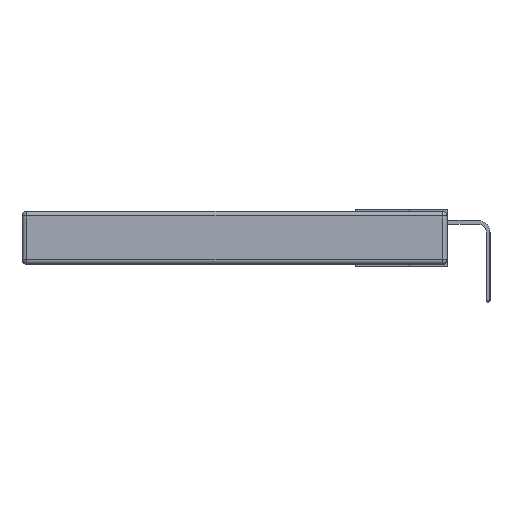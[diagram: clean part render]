
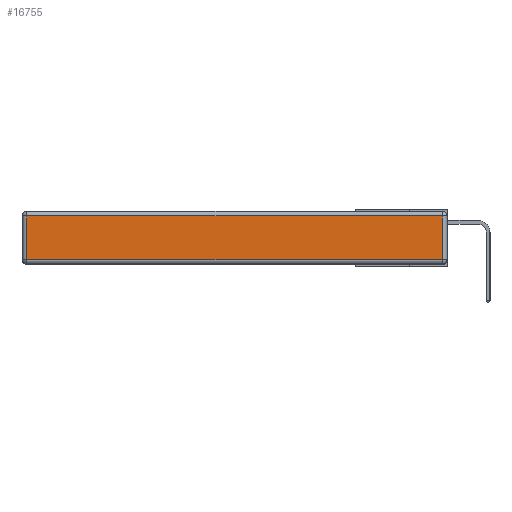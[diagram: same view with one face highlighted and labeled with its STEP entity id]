
A CAD part, left-side view. The second image highlights one B-rep face of the part: STEP entity #16755.
In plain terms, the highlighted planar face has unit normal (-1, 0, 0).
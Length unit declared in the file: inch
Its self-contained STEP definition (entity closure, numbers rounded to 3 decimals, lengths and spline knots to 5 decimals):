
#50 = ORIENTED_EDGE ( 'NONE', *, *, #7156, .T. ) ;
#140 = VECTOR ( 'NONE', #5073, 39.37008 ) ;
#407 = EDGE_LOOP ( 'NONE', ( #4328, #50, #971, #8789 ) ) ;
#781 = VERTEX_POINT ( 'NONE', #8965 ) ;
#971 = ORIENTED_EDGE ( 'NONE', *, *, #10357, .T. ) ;
#1026 = DIRECTION ( 'NONE',  ( 0., -1., 0. ) ) ;
#1210 = VERTEX_POINT ( 'NONE', #8549 ) ;
#1530 = FACE_OUTER_BOUND ( 'NONE', #407, .T. ) ;
#4133 = LINE ( 'NONE', #7741, #140 ) ;
#4328 = ORIENTED_EDGE ( 'NONE', *, *, #12384, .T. ) ;
#4814 = VECTOR ( 'NONE', #6618, 39.37008 ) ;
#5072 = VECTOR ( 'NONE', #11186, 39.37008 ) ;
#5073 = DIRECTION ( 'NONE',  ( 0., 1., 0. ) ) ;
#5142 = AXIS2_PLACEMENT_3D ( 'NONE', #17005, #18372, #6391 ) ;
#6391 = DIRECTION ( 'NONE',  ( 0., 0., 1. ) ) ;
#6618 = DIRECTION ( 'NONE',  ( 0., 0., 1. ) ) ;
#6680 = EDGE_CURVE ( 'NONE', #781, #11388, #12051, .T. ) ;
#7156 = EDGE_CURVE ( 'NONE', #1210, #17704, #12494, .T. ) ;
#7741 = CARTESIAN_POINT ( 'NONE',  ( 0., 2.75, -0.03 ) ) ;
#8190 = CARTESIAN_POINT ( 'NONE',  ( 0., 2.72, -0.343 ) ) ;
#8549 = CARTESIAN_POINT ( 'NONE',  ( 0., 0.03, -0.313 ) ) ;
#8789 = ORIENTED_EDGE ( 'NONE', *, *, #6680, .T. ) ;
#8965 = CARTESIAN_POINT ( 'NONE',  ( 0., 2.72, -0.03 ) ) ;
#9077 = CARTESIAN_POINT ( 'NONE',  ( 0., 2.72, -0.313 ) ) ;
#10357 = EDGE_CURVE ( 'NONE', #17704, #781, #4133, .T. ) ;
#11186 = DIRECTION ( 'NONE',  ( 0., 0., -1. ) ) ;
#11388 = VERTEX_POINT ( 'NONE', #9077 ) ;
#12051 = LINE ( 'NONE', #8190, #5072 ) ;
#12383 = PLANE ( 'NONE',  #5142 ) ;
#12384 = EDGE_CURVE ( 'NONE', #11388, #1210, #16413, .T. ) ;
#12494 = LINE ( 'NONE', #12741, #4814 ) ;
#12741 = CARTESIAN_POINT ( 'NONE',  ( 0., 0.03, -0.343 ) ) ;
#15970 = VECTOR ( 'NONE', #1026, 39.37008 ) ;
#16413 = LINE ( 'NONE', #17519, #15970 ) ;
#16755 = ADVANCED_FACE ( 'NONE', ( #1530 ), #12383, .T. ) ;
#17005 = CARTESIAN_POINT ( 'NONE',  ( 0., 0., -0.343 ) ) ;
#17034 = CARTESIAN_POINT ( 'NONE',  ( 0., 0.03, -0.03 ) ) ;
#17519 = CARTESIAN_POINT ( 'NONE',  ( 0., 0., -0.313 ) ) ;
#17704 = VERTEX_POINT ( 'NONE', #17034 ) ;
#18372 = DIRECTION ( 'NONE',  ( -1., 0., 0. ) ) ;
